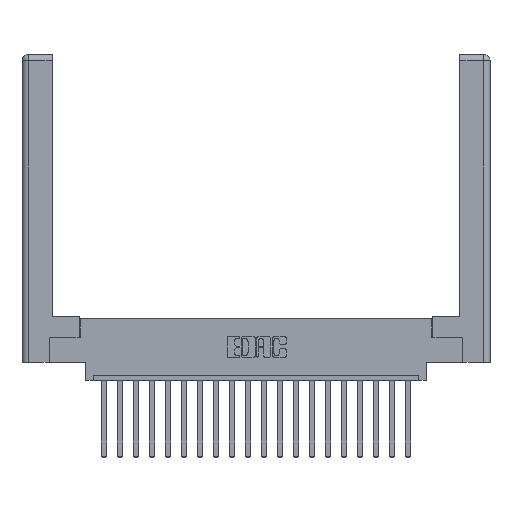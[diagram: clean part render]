
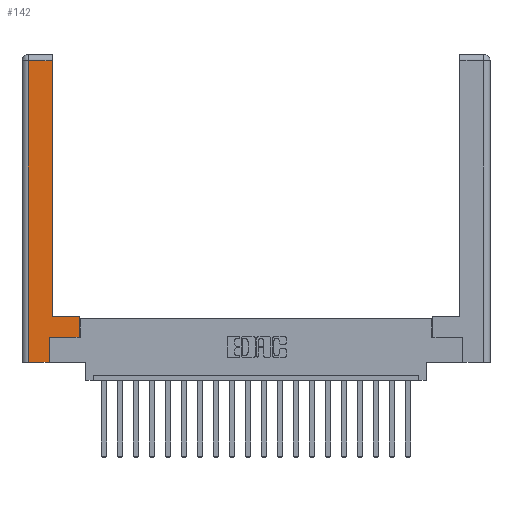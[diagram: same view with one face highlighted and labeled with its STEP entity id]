
A CAD part, top view. The second image highlights one B-rep face of the part: STEP entity #142.
In plain terms, the highlighted planar face has unit normal (0, 0, 1).
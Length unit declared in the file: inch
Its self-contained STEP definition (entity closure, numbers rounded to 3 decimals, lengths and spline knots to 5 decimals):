
#142 = ADVANCED_FACE ( 'NONE', ( #2305 ), #525, .F. ) ;
#188 = EDGE_CURVE ( 'NONE', #8849, #8352, #13342, .T. ) ;
#257 = LINE ( 'NONE', #7769, #11740 ) ;
#525 = PLANE ( 'NONE',  #19642 ) ;
#832 = EDGE_CURVE ( 'NONE', #14117, #12447, #13825, .T. ) ;
#1372 = ORIENTED_EDGE ( 'NONE', *, *, #7176, .T. ) ;
#1827 = CARTESIAN_POINT ( 'NONE',  ( 0.0615, 2.94, 0. ) ) ;
#2236 = DIRECTION ( 'NONE',  ( 1., 0., 0. ) ) ;
#2305 = FACE_OUTER_BOUND ( 'NONE', #15539, .T. ) ;
#2498 = ORIENTED_EDGE ( 'NONE', *, *, #6722, .T. ) ;
#2559 = CARTESIAN_POINT ( 'NONE',  ( 0.295, 2.94, 0. ) ) ;
#2744 = ORIENTED_EDGE ( 'NONE', *, *, #188, .T. ) ;
#3141 = VERTEX_POINT ( 'NONE', #6593 ) ;
#3683 = DIRECTION ( 'NONE',  ( 0., 0., -1. ) ) ;
#4585 = DIRECTION ( 'NONE',  ( 0., 1., 0. ) ) ;
#4615 = EDGE_CURVE ( 'NONE', #8352, #3141, #10697, .T. ) ;
#4924 = VERTEX_POINT ( 'NONE', #6434 ) ;
#5257 = LINE ( 'NONE', #8844, #18304 ) ;
#6192 = CARTESIAN_POINT ( 'NONE',  ( 0.0615, 2.94, 0. ) ) ;
#6434 = CARTESIAN_POINT ( 'NONE',  ( 0.265, 0.245, 0. ) ) ;
#6593 = CARTESIAN_POINT ( 'NONE',  ( 0.265, 0., 0. ) ) ;
#6702 = EDGE_CURVE ( 'NONE', #12447, #19712, #12239, .T. ) ;
#6722 = EDGE_CURVE ( 'NONE', #19712, #8849, #19141, .T. ) ;
#7176 = EDGE_CURVE ( 'NONE', #4924, #8032, #257, .T. ) ;
#7486 = VECTOR ( 'NONE', #7757, 39.37008 ) ;
#7690 = CARTESIAN_POINT ( 'NONE',  ( 0.265, 0.245, 0. ) ) ;
#7705 = DIRECTION ( 'NONE',  ( 1., 0., 0. ) ) ;
#7757 = DIRECTION ( 'NONE',  ( 0., 1., 0. ) ) ;
#7769 = CARTESIAN_POINT ( 'NONE',  ( 0.565, 0.245, 0. ) ) ;
#7845 = CARTESIAN_POINT ( 'NONE',  ( 0.295, 0.45, 0. ) ) ;
#7922 = ORIENTED_EDGE ( 'NONE', *, *, #16071, .T. ) ;
#7941 = VECTOR ( 'NONE', #11659, 39.37008 ) ;
#8032 = VERTEX_POINT ( 'NONE', #15022 ) ;
#8352 = VERTEX_POINT ( 'NONE', #16471 ) ;
#8844 = CARTESIAN_POINT ( 'NONE',  ( 0.565, 0.45, 0. ) ) ;
#8849 = VERTEX_POINT ( 'NONE', #6192 ) ;
#9813 = DIRECTION ( 'NONE',  ( -1., 0., 0. ) ) ;
#9976 = LINE ( 'NONE', #7690, #7486 ) ;
#10061 = ORIENTED_EDGE ( 'NONE', *, *, #6702, .T. ) ;
#10078 = CARTESIAN_POINT ( 'NONE',  ( 0.0615, 0., 0. ) ) ;
#10200 = VECTOR ( 'NONE', #2236, 39.37008 ) ;
#10697 = LINE ( 'NONE', #14748, #10200 ) ;
#10891 = VECTOR ( 'NONE', #11962, 39.37008 ) ;
#11232 = DIRECTION ( 'NONE',  ( 0., 1., 0. ) ) ;
#11259 = ORIENTED_EDGE ( 'NONE', *, *, #4615, .T. ) ;
#11659 = DIRECTION ( 'NONE',  ( 0., -1., 0. ) ) ;
#11740 = VECTOR ( 'NONE', #7705, 39.37008 ) ;
#11962 = DIRECTION ( 'NONE',  ( -1., 0., 0. ) ) ;
#11997 = VECTOR ( 'NONE', #18840, 39.37008 ) ;
#12239 = LINE ( 'NONE', #12883, #18133 ) ;
#12447 = VERTEX_POINT ( 'NONE', #7845 ) ;
#12883 = CARTESIAN_POINT ( 'NONE',  ( 0.295, 3., 0. ) ) ;
#13104 = CARTESIAN_POINT ( 'NONE',  ( 0., 0., 0. ) ) ;
#13342 = LINE ( 'NONE', #10078, #7941 ) ;
#13825 = LINE ( 'NONE', #15271, #10891 ) ;
#14117 = VERTEX_POINT ( 'NONE', #17188 ) ;
#14748 = CARTESIAN_POINT ( 'NONE',  ( 0.265, 0., 0. ) ) ;
#15022 = CARTESIAN_POINT ( 'NONE',  ( 0.565, 0.245, 0. ) ) ;
#15271 = CARTESIAN_POINT ( 'NONE',  ( 0.295, 0.45, 0. ) ) ;
#15539 = EDGE_LOOP ( 'NONE', ( #10061, #2498, #2744, #11259, #7922, #1372, #18947, #17294 ) ) ;
#16071 = EDGE_CURVE ( 'NONE', #3141, #4924, #9976, .T. ) ;
#16471 = CARTESIAN_POINT ( 'NONE',  ( 0.0615, 0., 0. ) ) ;
#16757 = EDGE_CURVE ( 'NONE', #8032, #14117, #5257, .T. ) ;
#17188 = CARTESIAN_POINT ( 'NONE',  ( 0.565, 0.45, 0. ) ) ;
#17294 = ORIENTED_EDGE ( 'NONE', *, *, #832, .T. ) ;
#18133 = VECTOR ( 'NONE', #11232, 39.37008 ) ;
#18304 = VECTOR ( 'NONE', #4585, 39.37008 ) ;
#18840 = DIRECTION ( 'NONE',  ( -1., 0., 0. ) ) ;
#18947 = ORIENTED_EDGE ( 'NONE', *, *, #16757, .T. ) ;
#19141 = LINE ( 'NONE', #1827, #11997 ) ;
#19642 = AXIS2_PLACEMENT_3D ( 'NONE', #13104, #3683, #9813 ) ;
#19712 = VERTEX_POINT ( 'NONE', #2559 ) ;
